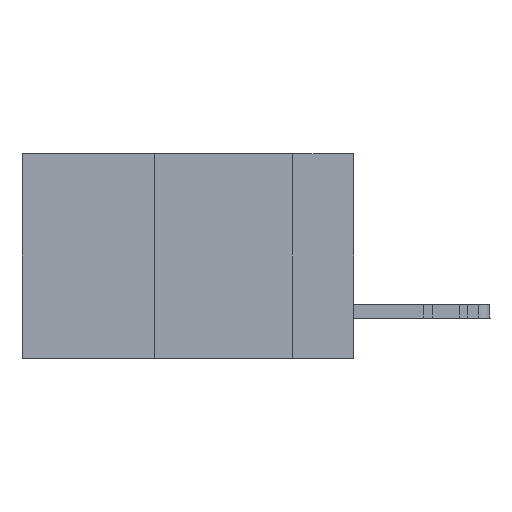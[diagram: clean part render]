
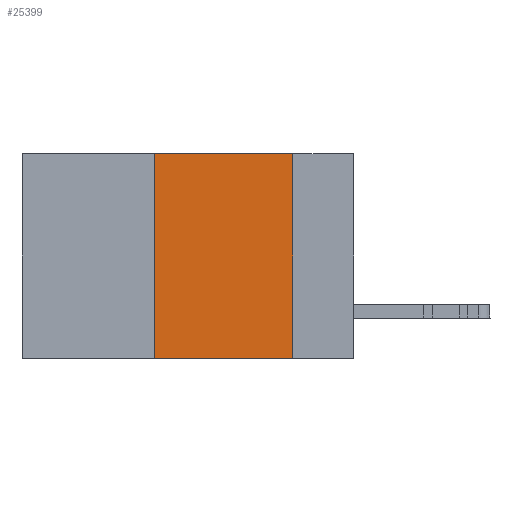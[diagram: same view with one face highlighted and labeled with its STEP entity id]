
A CAD part, left-side view. The second image highlights one B-rep face of the part: STEP entity #25399.
In plain terms, the highlighted planar face has unit normal (-1, 0, 0).
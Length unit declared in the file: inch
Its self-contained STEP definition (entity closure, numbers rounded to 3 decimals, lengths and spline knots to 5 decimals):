
#313 = VECTOR ( 'NONE', #36855, 39.37008 ) ;
#730 = CARTESIAN_POINT ( 'NONE',  ( 0., 0.11, 0. ) ) ;
#1812 = PLANE ( 'NONE',  #10366 ) ;
#2339 = LINE ( 'NONE', #27178, #27771 ) ;
#2395 = LINE ( 'NONE', #40094, #27833 ) ;
#3904 = CARTESIAN_POINT ( 'NONE',  ( 0., 0.36, 0. ) ) ;
#8099 = EDGE_CURVE ( 'NONE', #22977, #23281, #34667, .T. ) ;
#9706 = DIRECTION ( 'NONE',  ( 0., 0., -1. ) ) ;
#10366 = AXIS2_PLACEMENT_3D ( 'NONE', #29026, #17294, #13487 ) ;
#11804 = VERTEX_POINT ( 'NONE', #3904 ) ;
#12923 = ORIENTED_EDGE ( 'NONE', *, *, #38562, .T. ) ;
#12962 = CARTESIAN_POINT ( 'NONE',  ( 0., 0.6, -0.37 ) ) ;
#13487 = DIRECTION ( 'NONE',  ( 0., 0., -1. ) ) ;
#13993 = LINE ( 'NONE', #12962, #313 ) ;
#17294 = DIRECTION ( 'NONE',  ( 1., 0., 0. ) ) ;
#18357 = ORIENTED_EDGE ( 'NONE', *, *, #40975, .F. ) ;
#20907 = ORIENTED_EDGE ( 'NONE', *, *, #21571, .F. ) ;
#21571 = EDGE_CURVE ( 'NONE', #11804, #22977, #2395, .T. ) ;
#22977 = VERTEX_POINT ( 'NONE', #730 ) ;
#23281 = VERTEX_POINT ( 'NONE', #46301 ) ;
#24255 = FACE_OUTER_BOUND ( 'NONE', #26769, .T. ) ;
#25399 = ADVANCED_FACE ( 'NONE', ( #24255 ), #1812, .F. ) ;
#26769 = EDGE_LOOP ( 'NONE', ( #45366, #20907, #18357, #12923 ) ) ;
#27178 = CARTESIAN_POINT ( 'NONE',  ( 0., 0.36, 0. ) ) ;
#27771 = VECTOR ( 'NONE', #30831, 39.37008 ) ;
#27833 = VECTOR ( 'NONE', #44084, 39.37008 ) ;
#29026 = CARTESIAN_POINT ( 'NONE',  ( 0., 0.6, 0. ) ) ;
#30329 = CARTESIAN_POINT ( 'NONE',  ( 0., 0.36, -0.37 ) ) ;
#30831 = DIRECTION ( 'NONE',  ( 0., 0., 1. ) ) ;
#31459 = VERTEX_POINT ( 'NONE', #30329 ) ;
#32191 = VECTOR ( 'NONE', #9706, 39.37008 ) ;
#32757 = CARTESIAN_POINT ( 'NONE',  ( 0., 0.11, 0. ) ) ;
#34667 = LINE ( 'NONE', #32757, #32191 ) ;
#36855 = DIRECTION ( 'NONE',  ( 0., -1., 0. ) ) ;
#38562 = EDGE_CURVE ( 'NONE', #31459, #23281, #13993, .T. ) ;
#40094 = CARTESIAN_POINT ( 'NONE',  ( 0., 0.6, 0. ) ) ;
#40975 = EDGE_CURVE ( 'NONE', #31459, #11804, #2339, .T. ) ;
#44084 = DIRECTION ( 'NONE',  ( 0., -1., 0. ) ) ;
#45366 = ORIENTED_EDGE ( 'NONE', *, *, #8099, .F. ) ;
#46301 = CARTESIAN_POINT ( 'NONE',  ( 0., 0.11, -0.37 ) ) ;
